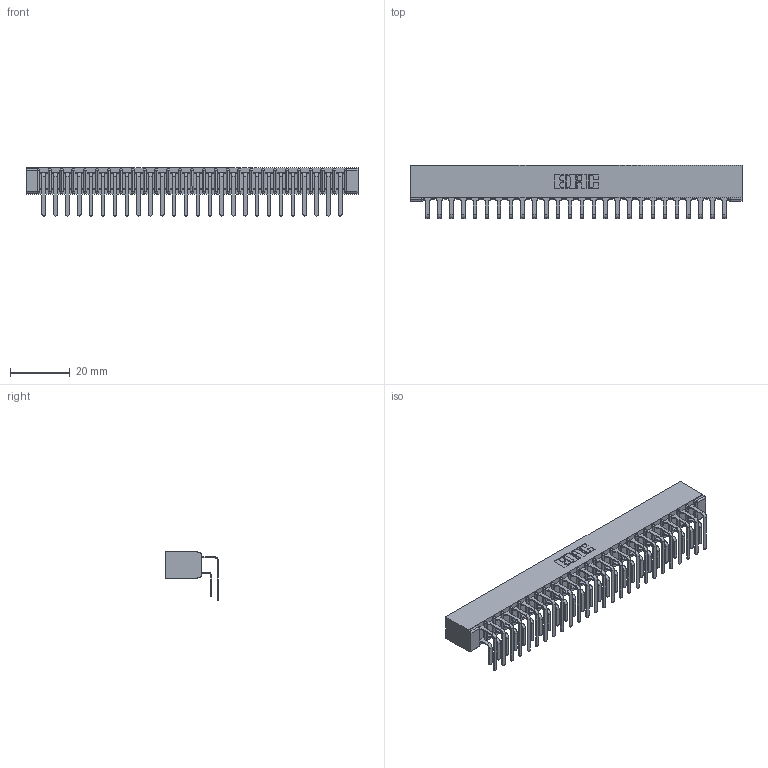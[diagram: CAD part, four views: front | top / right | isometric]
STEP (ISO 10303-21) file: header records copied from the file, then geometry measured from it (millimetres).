
FILE_DESCRIPTION (( 'STEP AP203' ), '1' );
FILE_NAME ('357-026-459-101.STEP', '2020-10-01T17:03:57', ( '' ), ( '' ), 'SwSTEP 2.0', 'SolidWorks 2020', '' );
FILE_SCHEMA (( 'CONFIG_CONTROL_DESIGN' ));
Length unit declared in the file: inch
Products named in the file (4): 307-290-001_558 559 - 1 (Single); 357-026-459-101; 307 Part_No Mounting Lugs; 307-290-001_559 - 2 (Single)
Assembly tree (53 placements, depth 2):
  357-026-459-101
    307 Part_No Mounting Lugs
    307-290-001_558 559 - 1 (Single)  x26
    307-290-001_559 - 2 (Single)  x26
Bounding box: 110.9 x 17.69 x 16.08 mm (x, y, z)
Volume: 7717 mm3; surface area: 15607.1 mm2
Topology: 53 solids, 53 shells, 2737 faces, 7683 edges, 4978 vertices
Faces by surface type: plane 1782, cylinder 901, sphere 54
Entity records: 26263 total; most frequent: CARTESIAN_POINT 4300, ORIENTED_EDGE 4258, DIRECTION 4217, EDGE_CURVE 2129, VECTOR 1627, LINE 1627, VERTEX_POINT 1378, AXIS2_PLACEMENT_3D 1295
